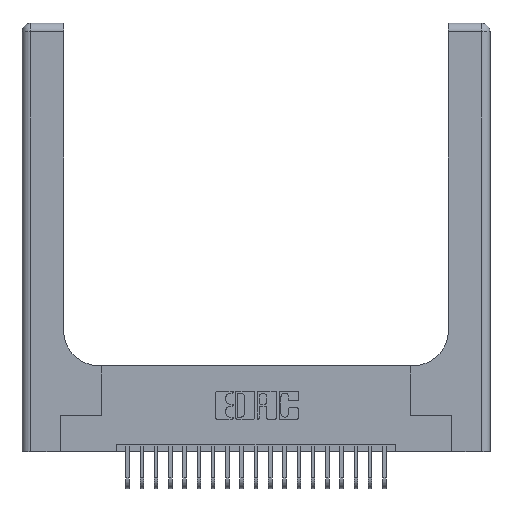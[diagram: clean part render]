
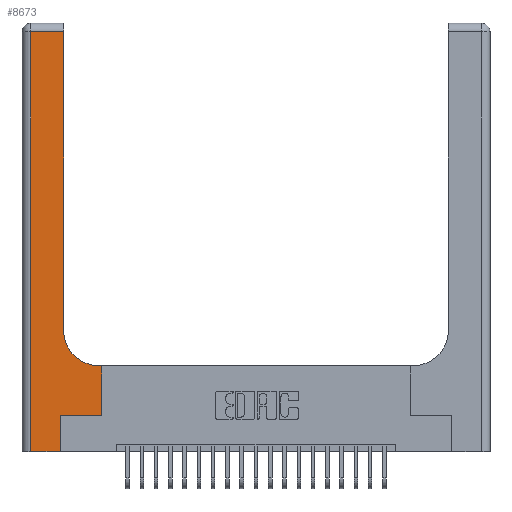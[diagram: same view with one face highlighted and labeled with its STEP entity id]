
A CAD part, top view. The second image highlights one B-rep face of the part: STEP entity #8673.
In plain terms, the highlighted planar face has unit normal (0, 0, 1).
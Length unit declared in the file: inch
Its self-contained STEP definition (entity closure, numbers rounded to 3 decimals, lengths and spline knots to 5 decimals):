
#656 = LINE ( 'NONE', #8834, #4766 ) ;
#762 = LINE ( 'NONE', #22432, #18785 ) ;
#1110 = VERTEX_POINT ( 'NONE', #15842 ) ;
#1342 = VERTEX_POINT ( 'NONE', #19861 ) ;
#1402 = DIRECTION ( 'NONE',  ( 1., 0., 0. ) ) ;
#1420 = CARTESIAN_POINT ( 'NONE',  ( 0.5415, 0.6, 0.37 ) ) ;
#1443 = PLANE ( 'NONE',  #20860 ) ;
#1462 = LINE ( 'NONE', #21107, #10232 ) ;
#1564 = ORIENTED_EDGE ( 'NONE', *, *, #19537, .T. ) ;
#2042 = ORIENTED_EDGE ( 'NONE', *, *, #3069, .T. ) ;
#2094 = EDGE_CURVE ( 'NONE', #1110, #17035, #12935, .T. ) ;
#2118 = AXIS2_PLACEMENT_3D ( 'NONE', #5718, #17898, #7486 ) ;
#2899 = LINE ( 'NONE', #9439, #12211 ) ;
#3069 = EDGE_CURVE ( 'NONE', #4587, #5638, #20832, .T. ) ;
#3078 = VECTOR ( 'NONE', #11464, 39.37008 ) ;
#3079 = CARTESIAN_POINT ( 'NONE',  ( 0.5585, 0.25, 0.37 ) ) ;
#3701 = LINE ( 'NONE', #11885, #16560 ) ;
#3831 = EDGE_CURVE ( 'NONE', #7859, #15942, #9604, .T. ) ;
#4587 = VERTEX_POINT ( 'NONE', #22659 ) ;
#4766 = VECTOR ( 'NONE', #21052, 39.37008 ) ;
#4946 = VECTOR ( 'NONE', #11879, 39.37008 ) ;
#4965 = DIRECTION ( 'NONE',  ( 0., 0., -1. ) ) ;
#5638 = VERTEX_POINT ( 'NONE', #6382 ) ;
#5718 = CARTESIAN_POINT ( 'NONE',  ( 0.5415, 0.85, 0.37 ) ) ;
#5803 = CARTESIAN_POINT ( 'NONE',  ( 0.269, 0.25, 0.37 ) ) ;
#6382 = CARTESIAN_POINT ( 'NONE',  ( 0.06, 2.94, 0.37 ) ) ;
#7486 = DIRECTION ( 'NONE',  ( 1., 0., 0. ) ) ;
#7545 = EDGE_CURVE ( 'NONE', #1342, #1110, #656, .T. ) ;
#7859 = VERTEX_POINT ( 'NONE', #11593 ) ;
#8183 = EDGE_CURVE ( 'NONE', #8695, #4587, #1462, .T. ) ;
#8673 = ADVANCED_FACE ( 'NONE', ( #18900 ), #1443, .F. ) ;
#8695 = VERTEX_POINT ( 'NONE', #13762 ) ;
#8834 = CARTESIAN_POINT ( 'NONE',  ( 0., 0., 0.37 ) ) ;
#8876 = DIRECTION ( 'NONE',  ( 0., 1., 0. ) ) ;
#9439 = CARTESIAN_POINT ( 'NONE',  ( 0.06, 3., 0.37 ) ) ;
#9447 = ORIENTED_EDGE ( 'NONE', *, *, #21507, .T. ) ;
#9468 = ORIENTED_EDGE ( 'NONE', *, *, #21723, .T. ) ;
#9604 = LINE ( 'NONE', #3079, #4946 ) ;
#10074 = VERTEX_POINT ( 'NONE', #1420 ) ;
#10232 = VECTOR ( 'NONE', #8876, 39.37008 ) ;
#10308 = DIRECTION ( 'NONE',  ( -1., 0., 0. ) ) ;
#11116 = DIRECTION ( 'NONE',  ( 0., -1., 0. ) ) ;
#11464 = DIRECTION ( 'NONE',  ( 0., 1., 0. ) ) ;
#11561 = VECTOR ( 'NONE', #15691, 39.37008 ) ;
#11593 = CARTESIAN_POINT ( 'NONE',  ( 0.5585, 0.25, 0.37 ) ) ;
#11879 = DIRECTION ( 'NONE',  ( 0., 1., 0. ) ) ;
#11885 = CARTESIAN_POINT ( 'NONE',  ( 0.269, 0.25, 0.37 ) ) ;
#12211 = VECTOR ( 'NONE', #11116, 39.37008 ) ;
#12729 = ORIENTED_EDGE ( 'NONE', *, *, #8183, .T. ) ;
#12884 = CARTESIAN_POINT ( 'NONE',  ( 0.5585, 0.6, 0.37 ) ) ;
#12935 = LINE ( 'NONE', #21917, #3078 ) ;
#13762 = CARTESIAN_POINT ( 'NONE',  ( 0.2915, 0.85, 0.37 ) ) ;
#15441 = CARTESIAN_POINT ( 'NONE',  ( 0., 3., 0.37 ) ) ;
#15473 = ORIENTED_EDGE ( 'NONE', *, *, #2094, .T. ) ;
#15691 = DIRECTION ( 'NONE',  ( -1., 0., 0. ) ) ;
#15842 = CARTESIAN_POINT ( 'NONE',  ( 0.269, 0., 0.37 ) ) ;
#15942 = VERTEX_POINT ( 'NONE', #12884 ) ;
#16560 = VECTOR ( 'NONE', #1402, 39.37008 ) ;
#17035 = VERTEX_POINT ( 'NONE', #5803 ) ;
#17166 = DIRECTION ( 'NONE',  ( -1., 0., 0. ) ) ;
#17352 = ORIENTED_EDGE ( 'NONE', *, *, #7545, .T. ) ;
#17659 = EDGE_CURVE ( 'NONE', #15942, #10074, #762, .T. ) ;
#17898 = DIRECTION ( 'NONE',  ( 0., 0., -1. ) ) ;
#18698 = EDGE_LOOP ( 'NONE', ( #12729, #2042, #9447, #17352, #15473, #9468, #22329, #21520, #1564 ) ) ;
#18785 = VECTOR ( 'NONE', #10308, 39.37008 ) ;
#18900 = FACE_OUTER_BOUND ( 'NONE', #18698, .T. ) ;
#19251 = CIRCLE ( 'NONE', #2118, 0.25 ) ;
#19537 = EDGE_CURVE ( 'NONE', #10074, #8695, #19251, .T. ) ;
#19861 = CARTESIAN_POINT ( 'NONE',  ( 0.06, 0., 0.37 ) ) ;
#20832 = LINE ( 'NONE', #20956, #11561 ) ;
#20860 = AXIS2_PLACEMENT_3D ( 'NONE', #15441, #4965, #17166 ) ;
#20956 = CARTESIAN_POINT ( 'NONE',  ( 0., 2.94, 0.37 ) ) ;
#21052 = DIRECTION ( 'NONE',  ( 1., 0., 0. ) ) ;
#21107 = CARTESIAN_POINT ( 'NONE',  ( 0.2915, 3., 0.37 ) ) ;
#21507 = EDGE_CURVE ( 'NONE', #5638, #1342, #2899, .T. ) ;
#21520 = ORIENTED_EDGE ( 'NONE', *, *, #17659, .T. ) ;
#21723 = EDGE_CURVE ( 'NONE', #17035, #7859, #3701, .T. ) ;
#21917 = CARTESIAN_POINT ( 'NONE',  ( 0.269, 0., 0.37 ) ) ;
#22329 = ORIENTED_EDGE ( 'NONE', *, *, #3831, .T. ) ;
#22432 = CARTESIAN_POINT ( 'NONE',  ( 0.2915, 0.6, 0.37 ) ) ;
#22659 = CARTESIAN_POINT ( 'NONE',  ( 0.2915, 2.94, 0.37 ) ) ;
